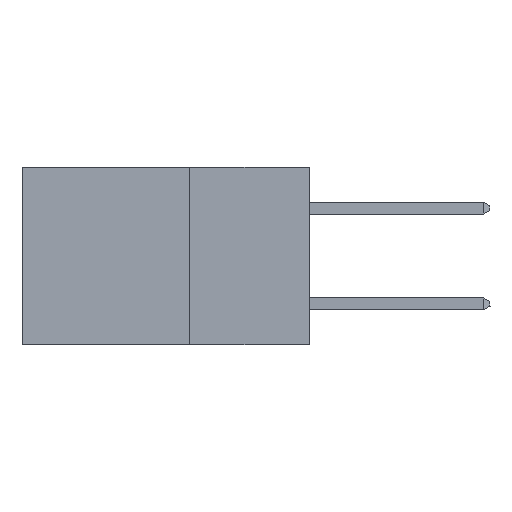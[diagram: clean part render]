
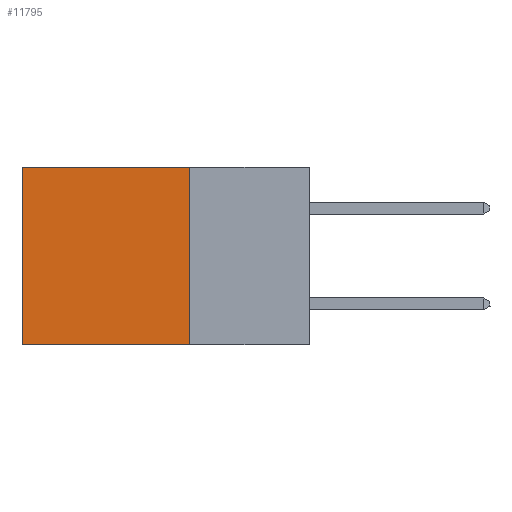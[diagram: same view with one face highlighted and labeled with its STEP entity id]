
A CAD part, left-side view. The second image highlights one B-rep face of the part: STEP entity #11795.
In plain terms, the highlighted planar face has unit normal (-1, 0, 0).
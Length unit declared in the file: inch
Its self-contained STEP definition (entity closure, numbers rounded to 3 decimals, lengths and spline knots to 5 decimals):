
#10 = VECTOR ( 'NONE', #15747, 39.37008 ) ;
#1494 = CARTESIAN_POINT ( 'NONE',  ( 0.2875, 0.25, -0.37 ) ) ;
#2832 = VERTEX_POINT ( 'NONE', #18222 ) ;
#3469 = EDGE_LOOP ( 'NONE', ( #19368, #6700, #4425, #21233 ) ) ;
#3503 = EDGE_CURVE ( 'NONE', #7231, #22323, #6559, .T. ) ;
#4425 = ORIENTED_EDGE ( 'NONE', *, *, #20000, .F. ) ;
#6311 = DIRECTION ( 'NONE',  ( 0., 1., 0. ) ) ;
#6559 = LINE ( 'NONE', #8112, #15549 ) ;
#6700 = ORIENTED_EDGE ( 'NONE', *, *, #3503, .F. ) ;
#7231 = VERTEX_POINT ( 'NONE', #1494 ) ;
#7960 = CARTESIAN_POINT ( 'NONE',  ( 0.2875, 0.25, 0. ) ) ;
#8112 = CARTESIAN_POINT ( 'NONE',  ( 0.2875, 0.25, -0.37 ) ) ;
#9717 = CARTESIAN_POINT ( 'NONE',  ( 0.2875, 0.25, 0. ) ) ;
#10269 = FACE_OUTER_BOUND ( 'NONE', #3469, .T. ) ;
#11795 = ADVANCED_FACE ( 'NONE', ( #10269 ), #13429, .F. ) ;
#13429 = PLANE ( 'NONE',  #14485 ) ;
#14485 = AXIS2_PLACEMENT_3D ( 'NONE', #9717, #26224, #18173 ) ;
#14985 = VERTEX_POINT ( 'NONE', #16130 ) ;
#15549 = VECTOR ( 'NONE', #6311, 39.37008 ) ;
#15574 = VECTOR ( 'NONE', #17613, 39.37008 ) ;
#15747 = DIRECTION ( 'NONE',  ( 0., 0., -1. ) ) ;
#16130 = CARTESIAN_POINT ( 'NONE',  ( 0.2875, 0.25, 0. ) ) ;
#17613 = DIRECTION ( 'NONE',  ( 0., 1., 0. ) ) ;
#17626 = CARTESIAN_POINT ( 'NONE',  ( 0.2875, 0.6, 0. ) ) ;
#17947 = EDGE_CURVE ( 'NONE', #2832, #22323, #21373, .T. ) ;
#18173 = DIRECTION ( 'NONE',  ( 0., 0., -1. ) ) ;
#18222 = CARTESIAN_POINT ( 'NONE',  ( 0.2875, 0.6, 0. ) ) ;
#19043 = CARTESIAN_POINT ( 'NONE',  ( 0.2875, 0.25, 0. ) ) ;
#19368 = ORIENTED_EDGE ( 'NONE', *, *, #17947, .T. ) ;
#19714 = EDGE_CURVE ( 'NONE', #14985, #2832, #26373, .T. ) ;
#20000 = EDGE_CURVE ( 'NONE', #14985, #7231, #24392, .T. ) ;
#20021 = VECTOR ( 'NONE', #22301, 39.37008 ) ;
#20579 = CARTESIAN_POINT ( 'NONE',  ( 0.2875, 0.6, -0.37 ) ) ;
#21233 = ORIENTED_EDGE ( 'NONE', *, *, #19714, .T. ) ;
#21373 = LINE ( 'NONE', #17626, #10 ) ;
#22301 = DIRECTION ( 'NONE',  ( 0., 0., -1. ) ) ;
#22323 = VERTEX_POINT ( 'NONE', #20579 ) ;
#24392 = LINE ( 'NONE', #7960, #20021 ) ;
#26224 = DIRECTION ( 'NONE',  ( 1., 0., 0. ) ) ;
#26373 = LINE ( 'NONE', #19043, #15574 ) ;
